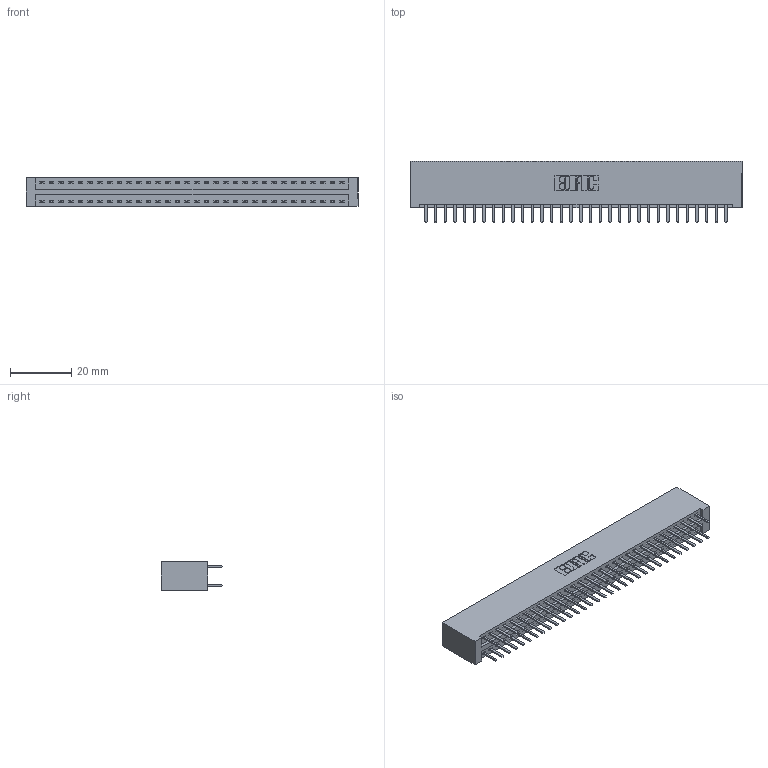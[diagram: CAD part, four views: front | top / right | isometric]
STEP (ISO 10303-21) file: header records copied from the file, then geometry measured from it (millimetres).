
FILE_DESCRIPTION (( 'STEP AP203' ), '1' );
FILE_NAME ('396-064-520-201.STEP', '2018-09-08T16:20:25', ( '' ), ( '' ), 'SwSTEP 2.0', 'SolidWorks 2016', '' );
FILE_SCHEMA (( 'CONFIG_CONTROL_DESIGN' ));
Length unit declared in the file: inch
Products named in the file (3): 396-064-520-201; 346 Part_No Mounting Lugs; 345-292-001_345-293-120
Assembly tree (65 placements, depth 2):
  396-064-520-201
    346 Part_No Mounting Lugs
    345-292-001_345-293-120  x64
Bounding box: 108.84 x 20.02 x 9.4 mm (x, y, z)
Volume: 11080.6 mm3; surface area: 15171.2 mm2
Topology: 65 solids, 65 shells, 3698 faces, 10737 edges, 6986 vertices
Faces by surface type: plane 2440, cylinder 1258
Entity records: 22067 total; most frequent: CARTESIAN_POINT 3660, ORIENTED_EDGE 3582, DIRECTION 3259, EDGE_CURVE 1791, VECTOR 1535, LINE 1535, VERTEX_POINT 1190, AXIS2_PLACEMENT_3D 862
